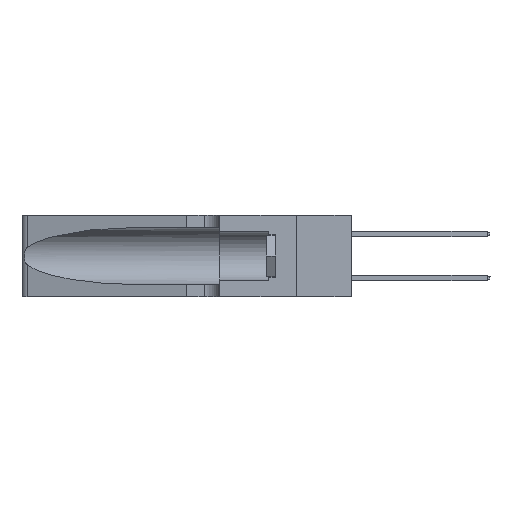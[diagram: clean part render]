
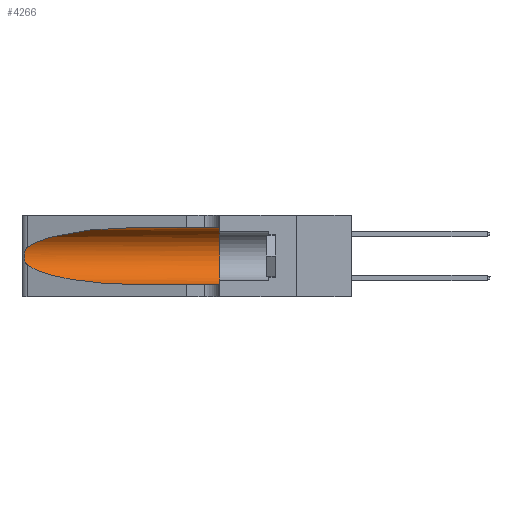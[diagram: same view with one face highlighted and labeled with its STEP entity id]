
A CAD part, left-side view. The second image highlights one B-rep face of the part: STEP entity #4266.
In plain terms, the highlighted cylindrical face has radius 3.308 mm (diameter 6.617 mm), a partial arc.
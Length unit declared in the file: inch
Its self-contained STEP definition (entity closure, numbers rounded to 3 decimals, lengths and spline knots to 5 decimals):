
#705 = DIRECTION ( 'NONE',  ( 0., -1., 0. ) ) ;
#790 = VERTEX_POINT ( 'NONE', #18415 ) ;
#1292 = EDGE_CURVE ( 'NONE', #790, #13565, #22074, .T. ) ;
#1349 = AXIS2_PLACEMENT_3D ( 'NONE', #8333, #8601, #6534 ) ;
#2864 = CARTESIAN_POINT ( 'NONE',  ( 0.2373, 1.15595, 0.28018 ) ) ;
#3833 = CARTESIAN_POINT ( 'NONE',  ( 0.1305, 0.72297, 0.05475 ) ) ;
#4266 = ADVANCED_FACE ( 'NONE', ( #7777 ), #23138, .F. ) ;
#4495 = CARTESIAN_POINT ( 'NONE',  ( 0.26075, 1.23896, 0.19203 ) ) ;
#4586 = CARTESIAN_POINT ( 'NONE',  ( 0.1305, 0.72297, 0.31525 ) ) ;
#4667 = CARTESIAN_POINT ( 'NONE',  ( 0.25487, 1.22718, 0.14631 ) ) ;
#4803 = VERTEX_POINT ( 'NONE', #15987 ) ;
#4999 = CIRCLE ( 'NONE', #1349, 0.13025 ) ;
#5132 = VERTEX_POINT ( 'NONE', #16819 ) ;
#5990 =( BOUNDED_CURVE ( )  B_SPLINE_CURVE ( 3, ( #21322, #17598, #13737, #3833 ),
 .UNSPECIFIED., .F., .T. ) 
 B_SPLINE_CURVE_WITH_KNOTS ( ( 4, 4 ),
 ( 3.44316, 4.71239 ),
 .UNSPECIFIED. ) 
 CURVE ( )  GEOMETRIC_REPRESENTATION_ITEM ( )  RATIONAL_B_SPLINE_CURVE ( ( 1., 0.87, 0.87, 1. ) ) 
 REPRESENTATION_ITEM ( '' )  );
#6119 = CARTESIAN_POINT ( 'NONE',  ( 0.25856, 1.23593, 0.16098 ) ) ;
#6534 = DIRECTION ( 'NONE',  ( 0., 0., 1. ) ) ;
#6577 = CARTESIAN_POINT ( 'NONE',  ( 0.25487, 1.22718, 0.22369 ) ) ;
#7493 = VECTOR ( 'NONE', #705, 39.37008 ) ;
#7556 = ORIENTED_EDGE ( 'NONE', *, *, #13909, .T. ) ;
#7777 = FACE_OUTER_BOUND ( 'NONE', #10993, .T. ) ;
#8333 = CARTESIAN_POINT ( 'NONE',  ( 0.1305, 0.35, 0.185 ) ) ;
#8533 = CARTESIAN_POINT ( 'NONE',  ( 0.1305, 1.61858, 0.31525 ) ) ;
#8601 = DIRECTION ( 'NONE',  ( 0., 1., 0. ) ) ;
#8680 = ORIENTED_EDGE ( 'NONE', *, *, #13951, .T. ) ;
#8941 = CARTESIAN_POINT ( 'NONE',  ( 0.26017, 1.23833, 0.17102 ) ) ;
#9232 = AXIS2_PLACEMENT_3D ( 'NONE', #9760, #11652, #15595 ) ;
#9643 = VERTEX_POINT ( 'NONE', #4586 ) ;
#9760 = CARTESIAN_POINT ( 'NONE',  ( 0.1305, 1.61858, 0.185 ) ) ;
#9927 = CARTESIAN_POINT ( 'NONE',  ( 0.25555, 1.22993, 0.14849 ) ) ;
#10595 = CARTESIAN_POINT ( 'NONE',  ( 0.26018, 1.23835, 0.19895 ) ) ;
#10615 = CARTESIAN_POINT ( 'NONE',  ( 0.26075, 1.23896, 0.178 ) ) ;
#10688 = ORIENTED_EDGE ( 'NONE', *, *, #17599, .F. ) ;
#10725 = CARTESIAN_POINT ( 'NONE',  ( 0.18966, 0.96281, 0.31525 ) ) ;
#10881 = CARTESIAN_POINT ( 'NONE',  ( 0.25639, 1.23184, 0.21858 ) ) ;
#10897 = CARTESIAN_POINT ( 'NONE',  ( 0.25639, 1.23186, 0.15144 ) ) ;
#10993 = EDGE_LOOP ( 'NONE', ( #24158, #21466, #8680, #7556, #10688, #17944 ) ) ;
#11652 = DIRECTION ( 'NONE',  ( 0., -1., 0. ) ) ;
#12693 = LINE ( 'NONE', #8533, #7493 ) ;
#12754 = CARTESIAN_POINT ( 'NONE',  ( 0.1305, 0.72297, 0.31525 ) ) ;
#12821 = CARTESIAN_POINT ( 'NONE',  ( 0.25787, 1.23484, 0.2124 ) ) ;
#13170 = LINE ( 'NONE', #13223, #15935 ) ;
#13223 = CARTESIAN_POINT ( 'NONE',  ( 0.1305, 1.61858, 0.05475 ) ) ;
#13340 = CARTESIAN_POINT ( 'NONE',  ( 0.25854, 1.2359, 0.20912 ) ) ;
#13565 = VERTEX_POINT ( 'NONE', #23940 ) ;
#13737 = CARTESIAN_POINT ( 'NONE',  ( 0.18966, 0.96281, 0.05475 ) ) ;
#13909 = EDGE_CURVE ( 'NONE', #21494, #4803, #13170, .T. ) ;
#13951 = EDGE_CURVE ( 'NONE', #13565, #21494, #5990, .T. ) ;
#15595 = DIRECTION ( 'NONE',  ( 0., 0., -1. ) ) ;
#15935 = VECTOR ( 'NONE', #16984, 39.37008 ) ;
#15987 = CARTESIAN_POINT ( 'NONE',  ( 0.1305, 0.35, 0.05475 ) ) ;
#16390 = EDGE_CURVE ( 'NONE', #9643, #790, #21316, .T. ) ;
#16819 = CARTESIAN_POINT ( 'NONE',  ( 0.1305, 0.35, 0.31525 ) ) ;
#16958 = EDGE_CURVE ( 'NONE', #9643, #5132, #12693, .T. ) ;
#16984 = DIRECTION ( 'NONE',  ( 0., -1., 0. ) ) ;
#17275 = CARTESIAN_POINT ( 'NONE',  ( 0.1305, 0.72297, 0.05475 ) ) ;
#17598 = CARTESIAN_POINT ( 'NONE',  ( 0.2373, 1.15595, 0.08982 ) ) ;
#17599 = EDGE_CURVE ( 'NONE', #5132, #4803, #4999, .T. ) ;
#17647 = CARTESIAN_POINT ( 'NONE',  ( 0.25789, 1.23486, 0.15765 ) ) ;
#17944 = ORIENTED_EDGE ( 'NONE', *, *, #16958, .F. ) ;
#18415 = CARTESIAN_POINT ( 'NONE',  ( 0.25487, 1.22718, 0.22369 ) ) ;
#20843 = CARTESIAN_POINT ( 'NONE',  ( 0.25487, 1.22718, 0.22369 ) ) ;
#21316 =( BOUNDED_CURVE ( )  B_SPLINE_CURVE ( 3, ( #12754, #10725, #2864, #20843 ),
 .UNSPECIFIED., .F., .F. ) 
 B_SPLINE_CURVE_WITH_KNOTS ( ( 4, 4 ),
 ( 1.5708, 2.84003 ),
 .UNSPECIFIED. ) 
 CURVE ( )  GEOMETRIC_REPRESENTATION_ITEM ( )  RATIONAL_B_SPLINE_CURVE ( ( 1., 0.87, 0.87, 1. ) ) 
 REPRESENTATION_ITEM ( '' )  );
#21322 = CARTESIAN_POINT ( 'NONE',  ( 0.25487, 1.22718, 0.14631 ) ) ;
#21466 = ORIENTED_EDGE ( 'NONE', *, *, #1292, .T. ) ;
#21494 = VERTEX_POINT ( 'NONE', #17275 ) ;
#22074 = B_SPLINE_CURVE_WITH_KNOTS ( 'NONE', 3,
 ( #6577, #24082, #10881, #12821, #13340, #10595, #4495, #10615, #8941, #6119, #17647, #10897, #9927, #4667 ),
 .UNSPECIFIED., .F., .F.,
 ( 4, 2, 2, 2, 2, 2, 4 ),
 ( 0., 0.00027, 0.00053, 0.00107, 0.0016, 0.00187, 0.00214 ),
 .UNSPECIFIED. ) ;
#23138 = CYLINDRICAL_SURFACE ( 'NONE', #9232, 0.13025 ) ;
#23940 = CARTESIAN_POINT ( 'NONE',  ( 0.25487, 1.22718, 0.14631 ) ) ;
#24082 = CARTESIAN_POINT ( 'NONE',  ( 0.25555, 1.22994, 0.2215 ) ) ;
#24158 = ORIENTED_EDGE ( 'NONE', *, *, #16390, .T. ) ;
